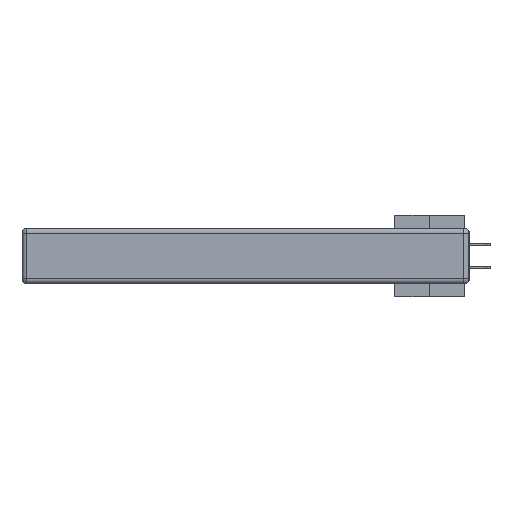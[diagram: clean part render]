
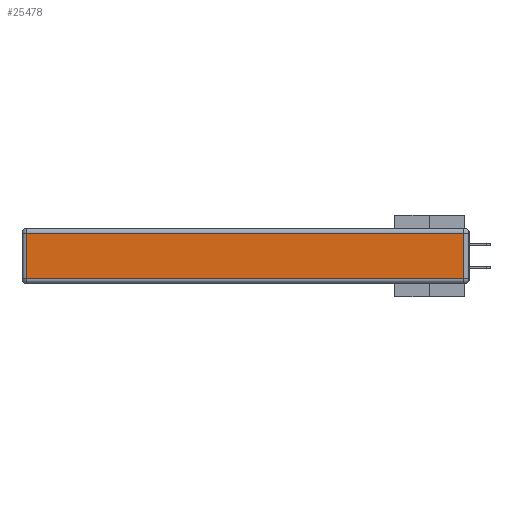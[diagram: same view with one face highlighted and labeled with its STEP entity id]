
A CAD part, left-side view. The second image highlights one B-rep face of the part: STEP entity #25478.
In plain terms, the highlighted planar face has unit normal (-1, 0, 0).
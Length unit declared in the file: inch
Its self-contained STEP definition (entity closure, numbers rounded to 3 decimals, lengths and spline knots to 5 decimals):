
#1255 = DIRECTION ( 'NONE',  ( 0., 0., -1. ) ) ;
#1258 = DIRECTION ( 'NONE',  ( -1., 0., 0. ) ) ;
#1261 = VECTOR ( 'NONE', #24019, 39.37008 ) ;
#3276 = LINE ( 'NONE', #36856, #1261 ) ;
#4121 = EDGE_CURVE ( 'NONE', #25472, #13336, #19449, .T. ) ;
#4547 = CARTESIAN_POINT ( 'NONE',  ( 0., 2.72, -0.343 ) ) ;
#7606 = ORIENTED_EDGE ( 'NONE', *, *, #4121, .T. ) ;
#7809 = CARTESIAN_POINT ( 'NONE',  ( 0., 0.03, -0.03 ) ) ;
#9234 = FACE_OUTER_BOUND ( 'NONE', #16274, .T. ) ;
#9281 = LINE ( 'NONE', #4547, #36376 ) ;
#10640 = ORIENTED_EDGE ( 'NONE', *, *, #23584, .T. ) ;
#10975 = AXIS2_PLACEMENT_3D ( 'NONE', #34381, #1258, #14830 ) ;
#11562 = PLANE ( 'NONE',  #10975 ) ;
#12425 = VERTEX_POINT ( 'NONE', #38439 ) ;
#13336 = VERTEX_POINT ( 'NONE', #38155 ) ;
#14830 = DIRECTION ( 'NONE',  ( 0., 0., 1. ) ) ;
#16178 = EDGE_CURVE ( 'NONE', #13336, #12425, #9281, .T. ) ;
#16274 = EDGE_LOOP ( 'NONE', ( #21624, #10640, #7606, #19515 ) ) ;
#19449 = LINE ( 'NONE', #26483, #27137 ) ;
#19515 = ORIENTED_EDGE ( 'NONE', *, *, #16178, .T. ) ;
#21624 = ORIENTED_EDGE ( 'NONE', *, *, #33026, .T. ) ;
#23584 = EDGE_CURVE ( 'NONE', #24093, #25472, #3276, .T. ) ;
#24019 = DIRECTION ( 'NONE',  ( 0., 0., 1. ) ) ;
#24093 = VERTEX_POINT ( 'NONE', #39314 ) ;
#25472 = VERTEX_POINT ( 'NONE', #7809 ) ;
#25478 = ADVANCED_FACE ( 'NONE', ( #9234 ), #11562, .T. ) ;
#26483 = CARTESIAN_POINT ( 'NONE',  ( 0., 2.75, -0.03 ) ) ;
#27137 = VECTOR ( 'NONE', #29617, 39.37008 ) ;
#29058 = VECTOR ( 'NONE', #38063, 39.37008 ) ;
#29617 = DIRECTION ( 'NONE',  ( 0., 1., 0. ) ) ;
#33026 = EDGE_CURVE ( 'NONE', #12425, #24093, #33677, .T. ) ;
#33677 = LINE ( 'NONE', #40244, #29058 ) ;
#34381 = CARTESIAN_POINT ( 'NONE',  ( 0., 0., -0.343 ) ) ;
#36376 = VECTOR ( 'NONE', #1255, 39.37008 ) ;
#36856 = CARTESIAN_POINT ( 'NONE',  ( 0., 0.03, -0.343 ) ) ;
#38063 = DIRECTION ( 'NONE',  ( 0., -1., 0. ) ) ;
#38155 = CARTESIAN_POINT ( 'NONE',  ( 0., 2.72, -0.03 ) ) ;
#38439 = CARTESIAN_POINT ( 'NONE',  ( 0., 2.72, -0.313 ) ) ;
#39314 = CARTESIAN_POINT ( 'NONE',  ( 0., 0.03, -0.313 ) ) ;
#40244 = CARTESIAN_POINT ( 'NONE',  ( 0., 0., -0.313 ) ) ;
